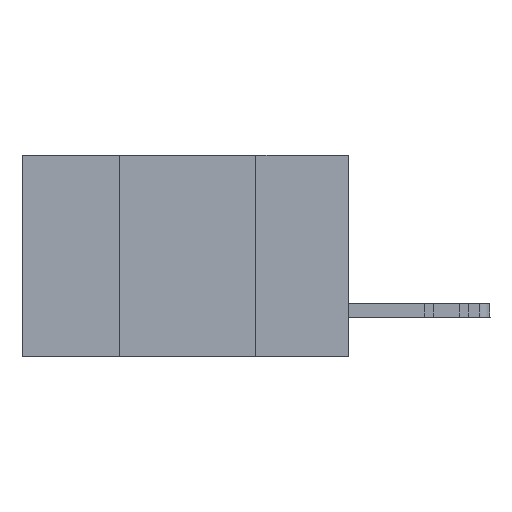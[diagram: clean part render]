
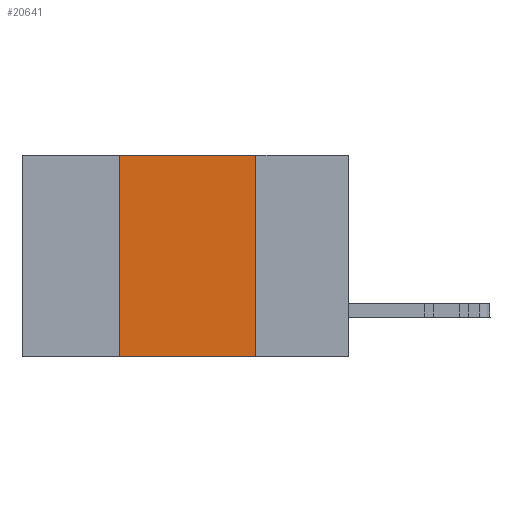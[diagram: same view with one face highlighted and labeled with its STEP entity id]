
A CAD part, left-side view. The second image highlights one B-rep face of the part: STEP entity #20641.
In plain terms, the highlighted planar face has unit normal (-1, 0, 0).
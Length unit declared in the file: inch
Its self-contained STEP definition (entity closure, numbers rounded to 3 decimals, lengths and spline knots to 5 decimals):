
#2046 = DIRECTION ( 'NONE',  ( 0., -1., 0. ) ) ;
#2371 = LINE ( 'NONE', #17526, #24431 ) ;
#2627 = VERTEX_POINT ( 'NONE', #24424 ) ;
#3173 = AXIS2_PLACEMENT_3D ( 'NONE', #16258, #11956, #27918 ) ;
#4197 = VECTOR ( 'NONE', #23121, 39.37008 ) ;
#5137 = EDGE_CURVE ( 'NONE', #14542, #2627, #2371, .T. ) ;
#5724 = VERTEX_POINT ( 'NONE', #11609 ) ;
#6330 = LINE ( 'NONE', #16539, #4197 ) ;
#7137 = LINE ( 'NONE', #21486, #25320 ) ;
#7393 = CARTESIAN_POINT ( 'NONE',  ( 0., 0.17, -0.37 ) ) ;
#9648 = CARTESIAN_POINT ( 'NONE',  ( 0., 0.42, 0. ) ) ;
#10050 = ORIENTED_EDGE ( 'NONE', *, *, #26544, .T. ) ;
#11013 = EDGE_CURVE ( 'NONE', #2627, #20642, #13101, .T. ) ;
#11609 = CARTESIAN_POINT ( 'NONE',  ( 0., 0.42, -0.37 ) ) ;
#11956 = DIRECTION ( 'NONE',  ( 1., 0., 0. ) ) ;
#13101 = LINE ( 'NONE', #23732, #24205 ) ;
#14542 = VERTEX_POINT ( 'NONE', #9648 ) ;
#16206 = EDGE_CURVE ( 'NONE', #5724, #14542, #7137, .T. ) ;
#16258 = CARTESIAN_POINT ( 'NONE',  ( 0., 0.6, 0. ) ) ;
#16539 = CARTESIAN_POINT ( 'NONE',  ( 0., 0.6, -0.37 ) ) ;
#16855 = FACE_OUTER_BOUND ( 'NONE', #18431, .T. ) ;
#16951 = DIRECTION ( 'NONE',  ( 0., 0., -1. ) ) ;
#17526 = CARTESIAN_POINT ( 'NONE',  ( 0., 0.6, 0. ) ) ;
#18431 = EDGE_LOOP ( 'NONE', ( #27594, #26876, #27334, #10050 ) ) ;
#20641 = ADVANCED_FACE ( 'NONE', ( #16855 ), #23334, .F. ) ;
#20642 = VERTEX_POINT ( 'NONE', #7393 ) ;
#21486 = CARTESIAN_POINT ( 'NONE',  ( 0., 0.42, 0. ) ) ;
#23121 = DIRECTION ( 'NONE',  ( 0., -1., 0. ) ) ;
#23334 = PLANE ( 'NONE',  #3173 ) ;
#23492 = DIRECTION ( 'NONE',  ( 0., 0., 1. ) ) ;
#23732 = CARTESIAN_POINT ( 'NONE',  ( 0., 0.17, 0. ) ) ;
#24205 = VECTOR ( 'NONE', #16951, 39.37008 ) ;
#24424 = CARTESIAN_POINT ( 'NONE',  ( 0., 0.17, 0. ) ) ;
#24431 = VECTOR ( 'NONE', #2046, 39.37008 ) ;
#25320 = VECTOR ( 'NONE', #23492, 39.37008 ) ;
#26544 = EDGE_CURVE ( 'NONE', #5724, #20642, #6330, .T. ) ;
#26876 = ORIENTED_EDGE ( 'NONE', *, *, #5137, .F. ) ;
#27334 = ORIENTED_EDGE ( 'NONE', *, *, #16206, .F. ) ;
#27594 = ORIENTED_EDGE ( 'NONE', *, *, #11013, .F. ) ;
#27918 = DIRECTION ( 'NONE',  ( 0., 0., -1. ) ) ;
